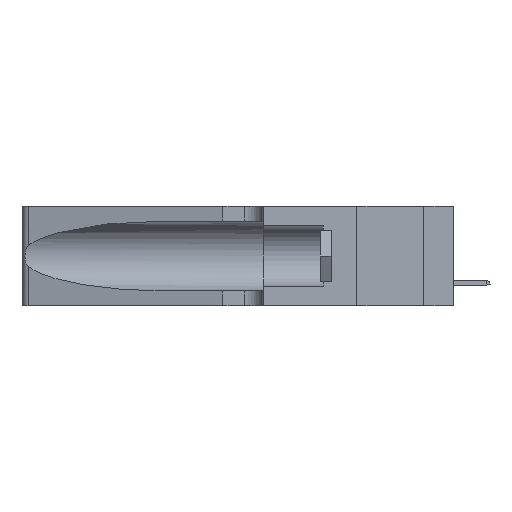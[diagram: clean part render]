
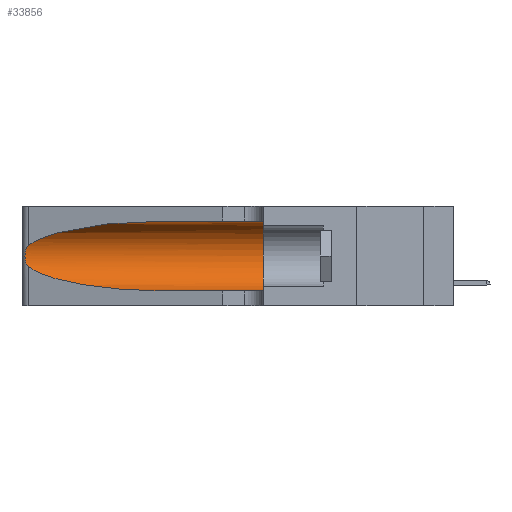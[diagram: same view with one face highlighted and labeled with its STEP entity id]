
A CAD part, left-side view. The second image highlights one B-rep face of the part: STEP entity #33856.
In plain terms, the highlighted cylindrical face has radius 3.308 mm (diameter 6.617 mm), a partial arc.
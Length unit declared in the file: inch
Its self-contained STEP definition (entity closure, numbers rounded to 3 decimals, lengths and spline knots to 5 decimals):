
#1478 = CARTESIAN_POINT ( 'NONE',  ( 0.2373, 1.15595, 0.08982 ) ) ;
#1651 =( BOUNDED_CURVE ( )  B_SPLINE_CURVE ( 3, ( #19409, #24909, #17299, #8770 ),
 .UNSPECIFIED., .F., .F. ) 
 B_SPLINE_CURVE_WITH_KNOTS ( ( 4, 4 ),
 ( 1.5708, 2.84003 ),
 .UNSPECIFIED. ) 
 CURVE ( )  GEOMETRIC_REPRESENTATION_ITEM ( )  RATIONAL_B_SPLINE_CURVE ( ( 1., 0.87, 0.87, 1. ) ) 
 REPRESENTATION_ITEM ( '' )  );
#3399 = CARTESIAN_POINT ( 'NONE',  ( 0.25487, 1.22718, 0.14631 ) ) ;
#4061 = CARTESIAN_POINT ( 'NONE',  ( 0.25487, 1.22718, 0.14631 ) ) ;
#4226 = CARTESIAN_POINT ( 'NONE',  ( 0.25854, 1.2359, 0.20912 ) ) ;
#4395 = CARTESIAN_POINT ( 'NONE',  ( 0.25787, 1.23484, 0.2124 ) ) ;
#4593 = DIRECTION ( 'NONE',  ( 0., 1., 0. ) ) ;
#4852 = B_SPLINE_CURVE_WITH_KNOTS ( 'NONE', 3,
 ( #7151, #25023, #17252, #4395, #4226, #33258, #25197, #12138, #15200, #17422, #31034, #22611, #12293, #4061 ),
 .UNSPECIFIED., .F., .F.,
 ( 4, 2, 2, 2, 2, 2, 4 ),
 ( 0., 0.00027, 0.00053, 0.00107, 0.0016, 0.00187, 0.00214 ),
 .UNSPECIFIED. ) ;
#6062 = AXIS2_PLACEMENT_3D ( 'NONE', #30895, #4593, #33132 ) ;
#6284 = CARTESIAN_POINT ( 'NONE',  ( 0.1305, 1.61858, 0.31525 ) ) ;
#6562 = VERTEX_POINT ( 'NONE', #28794 ) ;
#6692 = DIRECTION ( 'NONE',  ( 0., 0., -1. ) ) ;
#7151 = CARTESIAN_POINT ( 'NONE',  ( 0.25487, 1.22718, 0.22369 ) ) ;
#8169 = EDGE_CURVE ( 'NONE', #19867, #19102, #25181, .T. ) ;
#8770 = CARTESIAN_POINT ( 'NONE',  ( 0.25487, 1.22718, 0.22369 ) ) ;
#9452 = CYLINDRICAL_SURFACE ( 'NONE', #28761, 0.13025 ) ;
#9756 = ORIENTED_EDGE ( 'NONE', *, *, #8169, .F. ) ;
#11886 = CARTESIAN_POINT ( 'NONE',  ( 0.1305, 0.72297, 0.31525 ) ) ;
#11951 = CARTESIAN_POINT ( 'NONE',  ( 0.18966, 0.96281, 0.05475 ) ) ;
#12138 = CARTESIAN_POINT ( 'NONE',  ( 0.26075, 1.23896, 0.178 ) ) ;
#12293 = CARTESIAN_POINT ( 'NONE',  ( 0.25555, 1.22993, 0.14849 ) ) ;
#12935 = VECTOR ( 'NONE', #33084, 39.37008 ) ;
#13381 = EDGE_LOOP ( 'NONE', ( #15505, #20859, #29945, #19864, #30400, #9756 ) ) ;
#15043 = CARTESIAN_POINT ( 'NONE',  ( 0.1305, 1.61858, 0.05475 ) ) ;
#15200 = CARTESIAN_POINT ( 'NONE',  ( 0.26017, 1.23833, 0.17102 ) ) ;
#15505 = ORIENTED_EDGE ( 'NONE', *, *, #24021, .T. ) ;
#16977 = FACE_OUTER_BOUND ( 'NONE', #13381, .T. ) ;
#17252 = CARTESIAN_POINT ( 'NONE',  ( 0.25639, 1.23184, 0.21858 ) ) ;
#17260 = DIRECTION ( 'NONE',  ( 0., -1., 0. ) ) ;
#17299 = CARTESIAN_POINT ( 'NONE',  ( 0.2373, 1.15595, 0.28018 ) ) ;
#17422 = CARTESIAN_POINT ( 'NONE',  ( 0.25856, 1.23593, 0.16098 ) ) ;
#17431 = LINE ( 'NONE', #15043, #21591 ) ;
#17624 = VERTEX_POINT ( 'NONE', #19868 ) ;
#17641 = EDGE_CURVE ( 'NONE', #33459, #31211, #4852, .T. ) ;
#19102 = VERTEX_POINT ( 'NONE', #28438 ) ;
#19409 = CARTESIAN_POINT ( 'NONE',  ( 0.1305, 0.72297, 0.31525 ) ) ;
#19864 = ORIENTED_EDGE ( 'NONE', *, *, #32650, .T. ) ;
#19867 = VERTEX_POINT ( 'NONE', #11886 ) ;
#19868 = CARTESIAN_POINT ( 'NONE',  ( 0.1305, 0.35, 0.05475 ) ) ;
#20298 = CIRCLE ( 'NONE', #6062, 0.13025 ) ;
#20510 =( BOUNDED_CURVE ( )  B_SPLINE_CURVE ( 3, ( #30502, #1478, #11951, #30682 ),
 .UNSPECIFIED., .F., .F. ) 
 B_SPLINE_CURVE_WITH_KNOTS ( ( 4, 4 ),
 ( 3.44316, 4.71239 ),
 .UNSPECIFIED. ) 
 CURVE ( )  GEOMETRIC_REPRESENTATION_ITEM ( )  RATIONAL_B_SPLINE_CURVE ( ( 1., 0.87, 0.87, 1. ) ) 
 REPRESENTATION_ITEM ( '' )  );
#20859 = ORIENTED_EDGE ( 'NONE', *, *, #17641, .T. ) ;
#21591 = VECTOR ( 'NONE', #17260, 39.37008 ) ;
#22021 = CARTESIAN_POINT ( 'NONE',  ( 0.1305, 1.61858, 0.185 ) ) ;
#22055 = CARTESIAN_POINT ( 'NONE',  ( 0.25487, 1.22718, 0.22369 ) ) ;
#22611 = CARTESIAN_POINT ( 'NONE',  ( 0.25639, 1.23186, 0.15144 ) ) ;
#24021 = EDGE_CURVE ( 'NONE', #19867, #33459, #1651, .T. ) ;
#24909 = CARTESIAN_POINT ( 'NONE',  ( 0.18966, 0.96281, 0.31525 ) ) ;
#25023 = CARTESIAN_POINT ( 'NONE',  ( 0.25555, 1.22994, 0.2215 ) ) ;
#25181 = LINE ( 'NONE', #6284, #12935 ) ;
#25197 = CARTESIAN_POINT ( 'NONE',  ( 0.26075, 1.23896, 0.19203 ) ) ;
#26776 = EDGE_CURVE ( 'NONE', #31211, #6562, #20510, .T. ) ;
#27486 = DIRECTION ( 'NONE',  ( 0., -1., 0. ) ) ;
#27583 = EDGE_CURVE ( 'NONE', #19102, #17624, #20298, .T. ) ;
#28438 = CARTESIAN_POINT ( 'NONE',  ( 0.1305, 0.35, 0.31525 ) ) ;
#28761 = AXIS2_PLACEMENT_3D ( 'NONE', #22021, #27486, #6692 ) ;
#28794 = CARTESIAN_POINT ( 'NONE',  ( 0.1305, 0.72297, 0.05475 ) ) ;
#29945 = ORIENTED_EDGE ( 'NONE', *, *, #26776, .T. ) ;
#30400 = ORIENTED_EDGE ( 'NONE', *, *, #27583, .F. ) ;
#30502 = CARTESIAN_POINT ( 'NONE',  ( 0.25487, 1.22718, 0.14631 ) ) ;
#30682 = CARTESIAN_POINT ( 'NONE',  ( 0.1305, 0.72297, 0.05475 ) ) ;
#30895 = CARTESIAN_POINT ( 'NONE',  ( 0.1305, 0.35, 0.185 ) ) ;
#31034 = CARTESIAN_POINT ( 'NONE',  ( 0.25789, 1.23486, 0.15765 ) ) ;
#31211 = VERTEX_POINT ( 'NONE', #3399 ) ;
#32650 = EDGE_CURVE ( 'NONE', #6562, #17624, #17431, .T. ) ;
#33084 = DIRECTION ( 'NONE',  ( 0., -1., 0. ) ) ;
#33132 = DIRECTION ( 'NONE',  ( 0., 0., 1. ) ) ;
#33258 = CARTESIAN_POINT ( 'NONE',  ( 0.26018, 1.23835, 0.19895 ) ) ;
#33459 = VERTEX_POINT ( 'NONE', #22055 ) ;
#33856 = ADVANCED_FACE ( 'NONE', ( #16977 ), #9452, .F. ) ;
